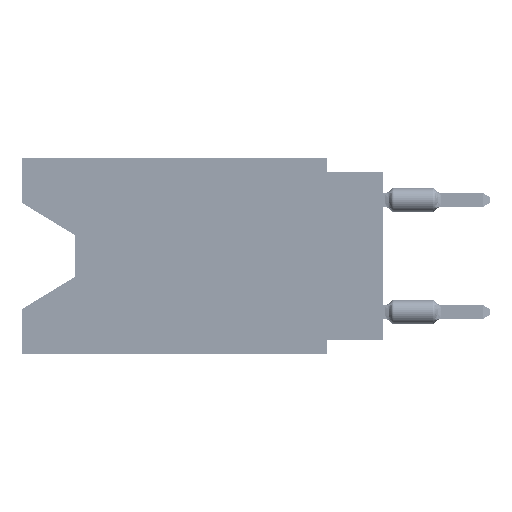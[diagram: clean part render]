
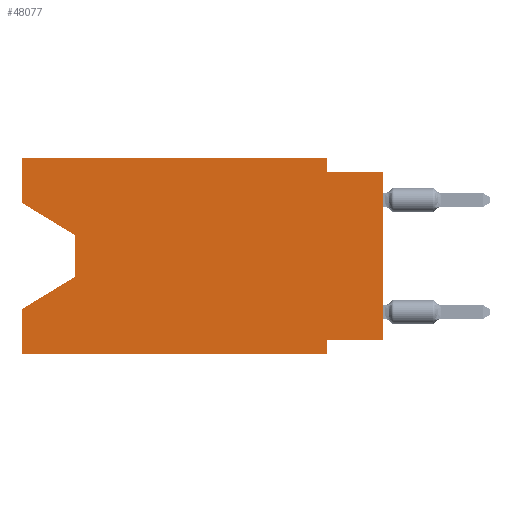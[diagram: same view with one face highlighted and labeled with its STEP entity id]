
A CAD part, left-side view. The second image highlights one B-rep face of the part: STEP entity #48077.
In plain terms, the highlighted planar face has unit normal (-1, 0, 0).
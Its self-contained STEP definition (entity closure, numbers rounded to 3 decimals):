
#136 = LINE ( 'NONE', #53313, #41142 ) ;
#854 = DIRECTION ( 'NONE',  ( 0., -1., 0. ) ) ;
#1514 = ORIENTED_EDGE ( 'NONE', *, *, #48328, .F. ) ;
#1554 = VECTOR ( 'NONE', #43706, 1000. ) ;
#2556 = CARTESIAN_POINT ( 'NONE',  ( 0., 0., -8.255 ) ) ;
#4079 = LINE ( 'NONE', #40002, #17967 ) ;
#5693 = CARTESIAN_POINT ( 'NONE',  ( 0., 16.383, 0. ) ) ;
#5771 = DIRECTION ( 'NONE',  ( 0., 0., 1. ) ) ;
#5929 = ORIENTED_EDGE ( 'NONE', *, *, #6298, .F. ) ;
#6035 = LINE ( 'NONE', #15224, #44794 ) ;
#6298 = EDGE_CURVE ( 'NONE', #23914, #43551, #24404, .T. ) ;
#6724 = ORIENTED_EDGE ( 'NONE', *, *, #40705, .T. ) ;
#7569 = ORIENTED_EDGE ( 'NONE', *, *, #34954, .F. ) ;
#7670 = FACE_OUTER_BOUND ( 'NONE', #54767, .T. ) ;
#7682 = ORIENTED_EDGE ( 'NONE', *, *, #16337, .F. ) ;
#9243 = CARTESIAN_POINT ( 'NONE',  ( 0., 13.97, -5.385 ) ) ;
#10038 = VECTOR ( 'NONE', #32472, 1000. ) ;
#10060 = CARTESIAN_POINT ( 'NONE',  ( 0., 16.383, 0. ) ) ;
#10133 = EDGE_CURVE ( 'NONE', #34859, #36898, #35580, .T. ) ;
#10451 = CARTESIAN_POINT ( 'NONE',  ( 0., 2.54, -8.255 ) ) ;
#10566 = LINE ( 'NONE', #14143, #23330 ) ;
#12183 = ORIENTED_EDGE ( 'NONE', *, *, #41435, .F. ) ;
#12563 = CARTESIAN_POINT ( 'NONE',  ( 0., 16.383, -8.89 ) ) ;
#12862 = VERTEX_POINT ( 'NONE', #48921 ) ;
#13856 = DIRECTION ( 'NONE',  ( 0., 0., 1. ) ) ;
#14056 = CARTESIAN_POINT ( 'NONE',  ( 0., 16.383, -8.89 ) ) ;
#14143 = CARTESIAN_POINT ( 'NONE',  ( 0., 2.54, 0. ) ) ;
#15224 = CARTESIAN_POINT ( 'NONE',  ( 0., 2.54, -8.89 ) ) ;
#16033 = AXIS2_PLACEMENT_3D ( 'NONE', #33820, #38849, #43881 ) ;
#16337 = EDGE_CURVE ( 'NONE', #36898, #20110, #6035, .T. ) ;
#17967 = VECTOR ( 'NONE', #13856, 1000. ) ;
#18637 = ORIENTED_EDGE ( 'NONE', *, *, #20202, .T. ) ;
#19257 = LINE ( 'NONE', #10060, #55642 ) ;
#19333 = VECTOR ( 'NONE', #27349, 1000. ) ;
#20110 = VERTEX_POINT ( 'NONE', #21446 ) ;
#20202 = EDGE_CURVE ( 'NONE', #12862, #46188, #53521, .T. ) ;
#21446 = CARTESIAN_POINT ( 'NONE',  ( 0., 2.54, -8.89 ) ) ;
#23112 = EDGE_CURVE ( 'NONE', #34859, #28500, #28045, .T. ) ;
#23330 = VECTOR ( 'NONE', #28684, 1000. ) ;
#23583 = CARTESIAN_POINT ( 'NONE',  ( 0., 0., 0. ) ) ;
#23914 = VERTEX_POINT ( 'NONE', #31402 ) ;
#24404 = LINE ( 'NONE', #33627, #50610 ) ;
#24768 = ORIENTED_EDGE ( 'NONE', *, *, #10133, .F. ) ;
#25769 = PLANE ( 'NONE',  #16033 ) ;
#26001 = DIRECTION ( 'NONE',  ( 0., -1., 0. ) ) ;
#27349 = DIRECTION ( 'NONE',  ( 0., 0.855, -0.519 ) ) ;
#27575 = ORIENTED_EDGE ( 'NONE', *, *, #23112, .T. ) ;
#28045 = LINE ( 'NONE', #23583, #29544 ) ;
#28500 = VERTEX_POINT ( 'NONE', #43303 ) ;
#28684 = DIRECTION ( 'NONE',  ( 0., 0., -1. ) ) ;
#28971 = VERTEX_POINT ( 'NONE', #12563 ) ;
#29544 = VECTOR ( 'NONE', #5771, 1000. ) ;
#30842 = DIRECTION ( 'NONE',  ( 0., 1., 0. ) ) ;
#31012 = EDGE_CURVE ( 'NONE', #53517, #12862, #37262, .T. ) ;
#31402 = CARTESIAN_POINT ( 'NONE',  ( 0., 16.383, -2.038 ) ) ;
#32472 = DIRECTION ( 'NONE',  ( 0., -1., 0. ) ) ;
#33109 = DIRECTION ( 'NONE',  ( 0., 0., -1. ) ) ;
#33267 = ORIENTED_EDGE ( 'NONE', *, *, #40582, .T. ) ;
#33627 = CARTESIAN_POINT ( 'NONE',  ( 0., 16.383, 0. ) ) ;
#33820 = CARTESIAN_POINT ( 'NONE',  ( 0., 16.383, 0. ) ) ;
#34859 = VERTEX_POINT ( 'NONE', #2556 ) ;
#34954 = EDGE_CURVE ( 'NONE', #49242, #28500, #136, .T. ) ;
#35009 = CARTESIAN_POINT ( 'NONE',  ( 0., 0., -8.255 ) ) ;
#35580 = LINE ( 'NONE', #35009, #46936 ) ;
#36453 = VERTEX_POINT ( 'NONE', #56566 ) ;
#36898 = VERTEX_POINT ( 'NONE', #10451 ) ;
#37262 = LINE ( 'NONE', #55664, #54989 ) ;
#37581 = EDGE_CURVE ( 'NONE', #36453, #49242, #10566, .T. ) ;
#38849 = DIRECTION ( 'NONE',  ( 1., 0., 0. ) ) ;
#40002 = CARTESIAN_POINT ( 'NONE',  ( 0., 16.383, 0. ) ) ;
#40582 = EDGE_CURVE ( 'NONE', #28971, #20110, #41665, .T. ) ;
#40705 = EDGE_CURVE ( 'NONE', #23914, #53517, #51748, .T. ) ;
#40992 = CARTESIAN_POINT ( 'NONE',  ( 0., 13.97, -3.505 ) ) ;
#41142 = VECTOR ( 'NONE', #26001, 1000. ) ;
#41435 = EDGE_CURVE ( 'NONE', #43551, #36453, #19257, .T. ) ;
#41665 = LINE ( 'NONE', #14056, #10038 ) ;
#43022 = CARTESIAN_POINT ( 'NONE',  ( 0., 2.54, -0.635 ) ) ;
#43303 = CARTESIAN_POINT ( 'NONE',  ( 0., 0., -0.635 ) ) ;
#43551 = VERTEX_POINT ( 'NONE', #5693 ) ;
#43706 = DIRECTION ( 'NONE',  ( 0., -0.855, -0.519 ) ) ;
#43881 = DIRECTION ( 'NONE',  ( 0., 0., -1. ) ) ;
#44794 = VECTOR ( 'NONE', #46977, 1000. ) ;
#46188 = VERTEX_POINT ( 'NONE', #54976 ) ;
#46936 = VECTOR ( 'NONE', #30842, 1000. ) ;
#46977 = DIRECTION ( 'NONE',  ( 0., 0., -1. ) ) ;
#48077 = ADVANCED_FACE ( 'NONE', ( #7670 ), #25769, .F. ) ;
#48328 = EDGE_CURVE ( 'NONE', #28971, #46188, #4079, .T. ) ;
#48921 = CARTESIAN_POINT ( 'NONE',  ( 0., 13.97, -5.385 ) ) ;
#49242 = VERTEX_POINT ( 'NONE', #43022 ) ;
#50610 = VECTOR ( 'NONE', #51427, 1000. ) ;
#51427 = DIRECTION ( 'NONE',  ( 0., 0., 1. ) ) ;
#51610 = ORIENTED_EDGE ( 'NONE', *, *, #37581, .F. ) ;
#51748 = LINE ( 'NONE', #52331, #1554 ) ;
#52331 = CARTESIAN_POINT ( 'NONE',  ( 0., 16.383, -2.038 ) ) ;
#52940 = ORIENTED_EDGE ( 'NONE', *, *, #31012, .T. ) ;
#53313 = CARTESIAN_POINT ( 'NONE',  ( 0., 0., -0.635 ) ) ;
#53517 = VERTEX_POINT ( 'NONE', #40992 ) ;
#53521 = LINE ( 'NONE', #9243, #19333 ) ;
#54767 = EDGE_LOOP ( 'NONE', ( #6724, #52940, #18637, #1514, #33267, #7682, #24768, #27575, #7569, #51610, #12183, #5929 ) ) ;
#54976 = CARTESIAN_POINT ( 'NONE',  ( 0., 16.383, -6.852 ) ) ;
#54989 = VECTOR ( 'NONE', #33109, 1000. ) ;
#55642 = VECTOR ( 'NONE', #854, 1000. ) ;
#55664 = CARTESIAN_POINT ( 'NONE',  ( 0., 13.97, -3.505 ) ) ;
#56566 = CARTESIAN_POINT ( 'NONE',  ( 0., 2.54, 0. ) ) ;
